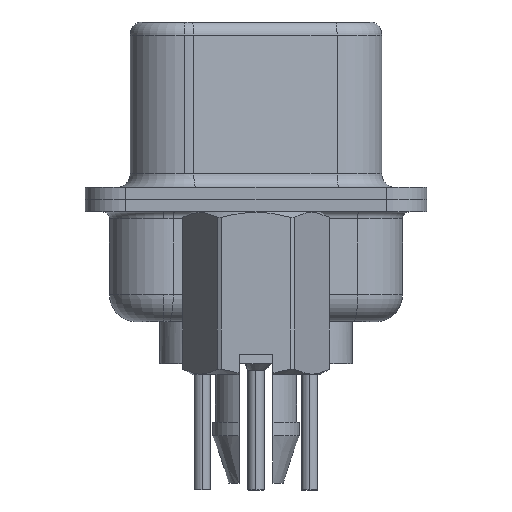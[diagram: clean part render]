
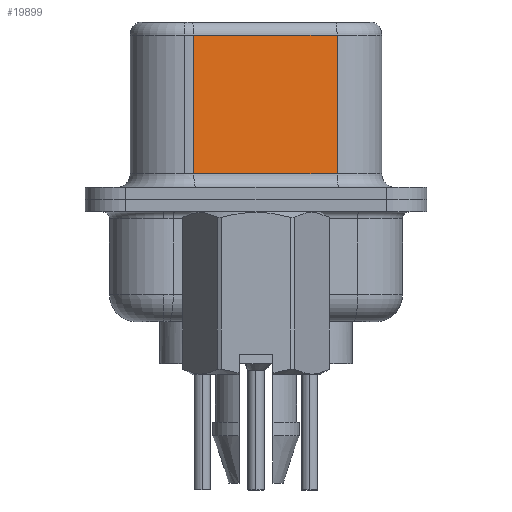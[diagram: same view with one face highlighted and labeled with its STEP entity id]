
A CAD part, left-side view. The second image highlights one B-rep face of the part: STEP entity #19899.
In plain terms, the highlighted planar face has unit normal (-0.985, -0.174, 0).
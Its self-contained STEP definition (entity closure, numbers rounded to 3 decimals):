
#577 = EDGE_CURVE ( 'NONE', #8207, #7477, #8642, .T. ) ;
#1364 = FACE_OUTER_BOUND ( 'NONE', #17897, .T. ) ;
#1874 = ORIENTED_EDGE ( 'NONE', *, *, #13134, .T. ) ;
#3151 = CARTESIAN_POINT ( 'NONE',  ( 3.615, 2.293, 6.57 ) ) ;
#3448 = AXIS2_PLACEMENT_3D ( 'NONE', #10635, #21377, #17302 ) ;
#3582 = DIRECTION ( 'NONE',  ( 0., 0., -1. ) ) ;
#4512 = VERTEX_POINT ( 'NONE', #23001 ) ;
#5141 = CARTESIAN_POINT ( 'NONE',  ( 3.615, 2.293, 0.95 ) ) ;
#5995 = LINE ( 'NONE', #12225, #10428 ) ;
#7477 = VERTEX_POINT ( 'NONE', #28187 ) ;
#8207 = VERTEX_POINT ( 'NONE', #5141 ) ;
#8642 = LINE ( 'NONE', #24281, #13119 ) ;
#9761 = EDGE_CURVE ( 'NONE', #4512, #12929, #5995, .T. ) ;
#9935 = ORIENTED_EDGE ( 'NONE', *, *, #9761, .T. ) ;
#10428 = VECTOR ( 'NONE', #19335, 1000. ) ;
#10503 = PLANE ( 'NONE',  #3448 ) ;
#10635 = CARTESIAN_POINT ( 'NONE',  ( 4.546, -2.987, 6.57 ) ) ;
#11606 = VECTOR ( 'NONE', #14428, 1000. ) ;
#12213 = ORIENTED_EDGE ( 'NONE', *, *, #14737, .F. ) ;
#12225 = CARTESIAN_POINT ( 'NONE',  ( 4.546, -2.987, 6.07 ) ) ;
#12929 = VERTEX_POINT ( 'NONE', #13592 ) ;
#12974 = VECTOR ( 'NONE', #3582, 1000. ) ;
#13119 = VECTOR ( 'NONE', #17191, 1000. ) ;
#13134 = EDGE_CURVE ( 'NONE', #12929, #8207, #14599, .T. ) ;
#13592 = CARTESIAN_POINT ( 'NONE',  ( 3.615, 2.293, 6.07 ) ) ;
#13925 = ORIENTED_EDGE ( 'NONE', *, *, #577, .T. ) ;
#14428 = DIRECTION ( 'NONE',  ( 0., 0., -1. ) ) ;
#14599 = LINE ( 'NONE', #3151, #12974 ) ;
#14737 = EDGE_CURVE ( 'NONE', #4512, #7477, #25140, .T. ) ;
#17191 = DIRECTION ( 'NONE',  ( 0.174, -0.985, 0. ) ) ;
#17302 = DIRECTION ( 'NONE',  ( -0.174, 0.985, 0. ) ) ;
#17897 = EDGE_LOOP ( 'NONE', ( #12213, #9935, #1874, #13925 ) ) ;
#19335 = DIRECTION ( 'NONE',  ( -0.174, 0.985, 0. ) ) ;
#19899 = ADVANCED_FACE ( 'NONE', ( #1364 ), #10503, .F. ) ;
#21377 = DIRECTION ( 'NONE',  ( 0.985, 0.174, 0. ) ) ;
#23001 = CARTESIAN_POINT ( 'NONE',  ( 4.546, -2.987, 6.07 ) ) ;
#24281 = CARTESIAN_POINT ( 'NONE',  ( 4.546, -2.987, 0.95 ) ) ;
#25140 = LINE ( 'NONE', #27587, #11606 ) ;
#27587 = CARTESIAN_POINT ( 'NONE',  ( 4.546, -2.987, 6.57 ) ) ;
#28187 = CARTESIAN_POINT ( 'NONE',  ( 4.546, -2.987, 0.95 ) ) ;
